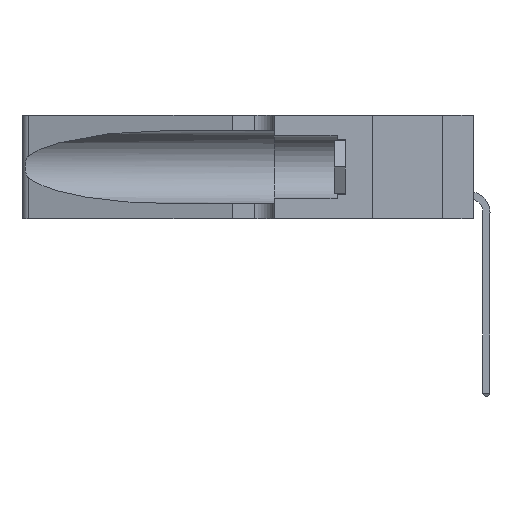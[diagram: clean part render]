
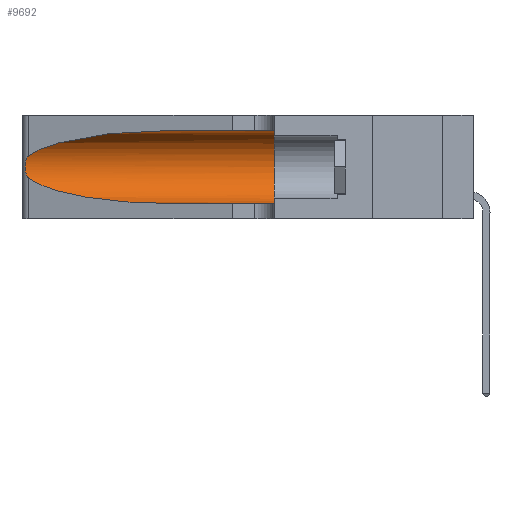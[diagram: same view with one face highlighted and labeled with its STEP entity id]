
A CAD part, left-side view. The second image highlights one B-rep face of the part: STEP entity #9692.
In plain terms, the highlighted cylindrical face has radius 3.308 mm (diameter 6.617 mm), a partial arc.
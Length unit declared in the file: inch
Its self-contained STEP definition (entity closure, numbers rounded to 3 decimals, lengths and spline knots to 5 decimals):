
#868 = CARTESIAN_POINT ( 'NONE',  ( 0.25555, 1.22993, 0.14849 ) ) ;
#1001 = CARTESIAN_POINT ( 'NONE',  ( 0.25487, 1.22718, 0.22369 ) ) ;
#1677 = DIRECTION ( 'NONE',  ( 0., 1., 0. ) ) ;
#2082 = CARTESIAN_POINT ( 'NONE',  ( 0.25487, 1.22718, 0.22369 ) ) ;
#3043 = VERTEX_POINT ( 'NONE', #2082 ) ;
#3059 = EDGE_CURVE ( 'NONE', #20815, #12802, #16570, .T. ) ;
#3220 = CARTESIAN_POINT ( 'NONE',  ( 0.25487, 1.22718, 0.22369 ) ) ;
#4946 = CARTESIAN_POINT ( 'NONE',  ( 0.1305, 0.72297, 0.31525 ) ) ;
#5542 = VERTEX_POINT ( 'NONE', #35656 ) ;
#6265 = AXIS2_PLACEMENT_3D ( 'NONE', #25583, #17965, #12868 ) ;
#6428 = EDGE_LOOP ( 'NONE', ( #13409, #17763, #27264, #27031, #31485, #29152 ) ) ;
#6909 = CARTESIAN_POINT ( 'NONE',  ( 0.26017, 1.23833, 0.17102 ) ) ;
#7145 = DIRECTION ( 'NONE',  ( 0., -1., 0. ) ) ;
#7148 = CARTESIAN_POINT ( 'NONE',  ( 0.25487, 1.22718, 0.14631 ) ) ;
#7859 = CARTESIAN_POINT ( 'NONE',  ( 0.1305, 0.72297, 0.05475 ) ) ;
#9154 = LINE ( 'NONE', #23754, #10038 ) ;
#9692 = ADVANCED_FACE ( 'NONE', ( #24196 ), #30268, .F. ) ;
#9700 = CARTESIAN_POINT ( 'NONE',  ( 0.26018, 1.23835, 0.19895 ) ) ;
#10038 = VECTOR ( 'NONE', #7145, 39.37008 ) ;
#10622 = DIRECTION ( 'NONE',  ( 0., -1., 0. ) ) ;
#11982 = CARTESIAN_POINT ( 'NONE',  ( 0.25639, 1.23184, 0.21858 ) ) ;
#12240 = CARTESIAN_POINT ( 'NONE',  ( 0.26075, 1.23896, 0.178 ) ) ;
#12802 = VERTEX_POINT ( 'NONE', #26615 ) ;
#12868 = DIRECTION ( 'NONE',  ( 0., 0., -1. ) ) ;
#13409 = ORIENTED_EDGE ( 'NONE', *, *, #26609, .T. ) ;
#15035 = CARTESIAN_POINT ( 'NONE',  ( 0.25789, 1.23486, 0.15765 ) ) ;
#15452 = DIRECTION ( 'NONE',  ( 0., 0., 1. ) ) ;
#16569 = EDGE_CURVE ( 'NONE', #12802, #25070, #16791, .T. ) ;
#16570 = LINE ( 'NONE', #21317, #33910 ) ;
#16791 = CIRCLE ( 'NONE', #27314, 0.13025 ) ;
#17763 = ORIENTED_EDGE ( 'NONE', *, *, #26731, .T. ) ;
#17965 = DIRECTION ( 'NONE',  ( 0., -1., 0. ) ) ;
#20341 = CARTESIAN_POINT ( 'NONE',  ( 0.26075, 1.23896, 0.19203 ) ) ;
#20467 = CARTESIAN_POINT ( 'NONE',  ( 0.25854, 1.2359, 0.20912 ) ) ;
#20595 = CARTESIAN_POINT ( 'NONE',  ( 0.25787, 1.23484, 0.2124 ) ) ;
#20815 = VERTEX_POINT ( 'NONE', #4946 ) ;
#21317 = CARTESIAN_POINT ( 'NONE',  ( 0.1305, 1.61858, 0.31525 ) ) ;
#21334 = CARTESIAN_POINT ( 'NONE',  ( 0.2373, 1.15595, 0.08982 ) ) ;
#22790 = CARTESIAN_POINT ( 'NONE',  ( 0.18966, 0.96281, 0.31525 ) ) ;
#23028 = CARTESIAN_POINT ( 'NONE',  ( 0.25487, 1.22718, 0.14631 ) ) ;
#23155 = CARTESIAN_POINT ( 'NONE',  ( 0.25856, 1.23593, 0.16098 ) ) ;
#23524 = CARTESIAN_POINT ( 'NONE',  ( 0.25555, 1.22994, 0.2215 ) ) ;
#23754 = CARTESIAN_POINT ( 'NONE',  ( 0.1305, 1.61858, 0.05475 ) ) ;
#24196 = FACE_OUTER_BOUND ( 'NONE', #6428, .T. ) ;
#24233 = CARTESIAN_POINT ( 'NONE',  ( 0.1305, 0.35, 0.05475 ) ) ;
#25070 = VERTEX_POINT ( 'NONE', #24233 ) ;
#25129 = VERTEX_POINT ( 'NONE', #7148 ) ;
#25583 = CARTESIAN_POINT ( 'NONE',  ( 0.1305, 1.61858, 0.185 ) ) ;
#26609 = EDGE_CURVE ( 'NONE', #20815, #3043, #30537, .T. ) ;
#26615 = CARTESIAN_POINT ( 'NONE',  ( 0.1305, 0.35, 0.31525 ) ) ;
#26731 = EDGE_CURVE ( 'NONE', #3043, #25129, #34327, .T. ) ;
#27031 = ORIENTED_EDGE ( 'NONE', *, *, #30382, .T. ) ;
#27264 = ORIENTED_EDGE ( 'NONE', *, *, #32237, .T. ) ;
#27314 = AXIS2_PLACEMENT_3D ( 'NONE', #29003, #1677, #15452 ) ;
#28012 = CARTESIAN_POINT ( 'NONE',  ( 0.2373, 1.15595, 0.28018 ) ) ;
#28117 = CARTESIAN_POINT ( 'NONE',  ( 0.1305, 0.72297, 0.31525 ) ) ;
#28310 =( BOUNDED_CURVE ( )  B_SPLINE_CURVE ( 3, ( #35473, #21334, #32463, #7859 ),
 .UNSPECIFIED., .F., .T. ) 
 B_SPLINE_CURVE_WITH_KNOTS ( ( 4, 4 ),
 ( 3.44316, 4.71239 ),
 .UNSPECIFIED. ) 
 CURVE ( )  GEOMETRIC_REPRESENTATION_ITEM ( )  RATIONAL_B_SPLINE_CURVE ( ( 1., 0.87, 0.87, 1. ) ) 
 REPRESENTATION_ITEM ( '' )  );
#29003 = CARTESIAN_POINT ( 'NONE',  ( 0.1305, 0.35, 0.185 ) ) ;
#29152 = ORIENTED_EDGE ( 'NONE', *, *, #3059, .F. ) ;
#30268 = CYLINDRICAL_SURFACE ( 'NONE', #6265, 0.13025 ) ;
#30382 = EDGE_CURVE ( 'NONE', #5542, #25070, #9154, .T. ) ;
#30537 =( BOUNDED_CURVE ( )  B_SPLINE_CURVE ( 3, ( #28117, #22790, #28012, #3220 ),
 .UNSPECIFIED., .F., .F. ) 
 B_SPLINE_CURVE_WITH_KNOTS ( ( 4, 4 ),
 ( 1.5708, 2.84003 ),
 .UNSPECIFIED. ) 
 CURVE ( )  GEOMETRIC_REPRESENTATION_ITEM ( )  RATIONAL_B_SPLINE_CURVE ( ( 1., 0.87, 0.87, 1. ) ) 
 REPRESENTATION_ITEM ( '' )  );
#31260 = CARTESIAN_POINT ( 'NONE',  ( 0.25639, 1.23186, 0.15144 ) ) ;
#31485 = ORIENTED_EDGE ( 'NONE', *, *, #16569, .F. ) ;
#32237 = EDGE_CURVE ( 'NONE', #25129, #5542, #28310, .T. ) ;
#32463 = CARTESIAN_POINT ( 'NONE',  ( 0.18966, 0.96281, 0.05475 ) ) ;
#33910 = VECTOR ( 'NONE', #10622, 39.37008 ) ;
#34327 = B_SPLINE_CURVE_WITH_KNOTS ( 'NONE', 3,
 ( #1001, #23524, #11982, #20595, #20467, #9700, #20341, #12240, #6909, #23155, #15035, #31260, #868, #23028 ),
 .UNSPECIFIED., .F., .F.,
 ( 4, 2, 2, 2, 2, 2, 4 ),
 ( 0., 0.00027, 0.00053, 0.00107, 0.0016, 0.00187, 0.00214 ),
 .UNSPECIFIED. ) ;
#35473 = CARTESIAN_POINT ( 'NONE',  ( 0.25487, 1.22718, 0.14631 ) ) ;
#35656 = CARTESIAN_POINT ( 'NONE',  ( 0.1305, 0.72297, 0.05475 ) ) ;
